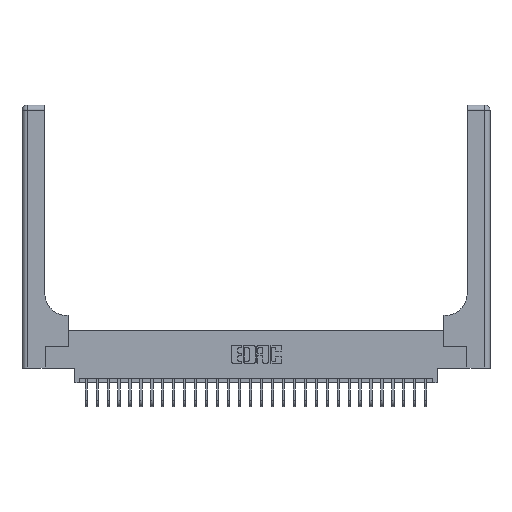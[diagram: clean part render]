
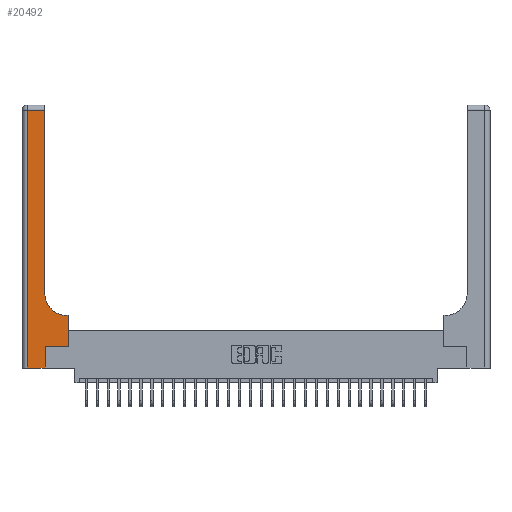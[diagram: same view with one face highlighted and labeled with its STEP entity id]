
A CAD part, top view. The second image highlights one B-rep face of the part: STEP entity #20492.
In plain terms, the highlighted planar face has unit normal (0, 0, 1).
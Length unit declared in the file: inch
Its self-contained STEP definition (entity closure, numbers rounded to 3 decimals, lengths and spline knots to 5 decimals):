
#137 = VERTEX_POINT ( 'NONE', #9777 ) ;
#267 = EDGE_LOOP ( 'NONE', ( #6003, #9272, #13486, #5783, #15114, #22827, #4643, #26591, #8260 ) ) ;
#576 = VERTEX_POINT ( 'NONE', #17336 ) ;
#908 = VECTOR ( 'NONE', #13147, 39.37008 ) ;
#946 = EDGE_CURVE ( 'NONE', #10002, #137, #17527, .T. ) ;
#1203 = CARTESIAN_POINT ( 'NONE',  ( 0.26, 2.94, 0.37 ) ) ;
#1216 = LINE ( 'NONE', #3422, #10927 ) ;
#1313 = PLANE ( 'NONE',  #22384 ) ;
#1940 = DIRECTION ( 'NONE',  ( -1., 0., 0. ) ) ;
#2091 = DIRECTION ( 'NONE',  ( 1., 0., 0. ) ) ;
#2163 = CARTESIAN_POINT ( 'NONE',  ( 0.51, 0.6, 0.37 ) ) ;
#2809 = LINE ( 'NONE', #24701, #23362 ) ;
#3154 = VECTOR ( 'NONE', #19565, 39.37008 ) ;
#3422 = CARTESIAN_POINT ( 'NONE',  ( 0., 0., 0.37 ) ) ;
#3699 = CARTESIAN_POINT ( 'NONE',  ( 0.528, 0.25, 0.37 ) ) ;
#4643 = ORIENTED_EDGE ( 'NONE', *, *, #16087, .T. ) ;
#5032 = VERTEX_POINT ( 'NONE', #20788 ) ;
#5483 = CARTESIAN_POINT ( 'NONE',  ( 0., 3., 0.37 ) ) ;
#5504 = DIRECTION ( 'NONE',  ( 1., 0., 0. ) ) ;
#5783 = ORIENTED_EDGE ( 'NONE', *, *, #23044, .T. ) ;
#5808 = CARTESIAN_POINT ( 'NONE',  ( 0.06, 2.94, 0.37 ) ) ;
#6003 = ORIENTED_EDGE ( 'NONE', *, *, #11436, .T. ) ;
#6098 = EDGE_CURVE ( 'NONE', #9677, #18002, #18338, .T. ) ;
#8156 = VERTEX_POINT ( 'NONE', #16663 ) ;
#8260 = ORIENTED_EDGE ( 'NONE', *, *, #946, .T. ) ;
#8759 = CARTESIAN_POINT ( 'NONE',  ( 0.265, 0.25, 0.37 ) ) ;
#8879 = LINE ( 'NONE', #11982, #19076 ) ;
#9272 = ORIENTED_EDGE ( 'NONE', *, *, #6098, .T. ) ;
#9677 = VERTEX_POINT ( 'NONE', #1203 ) ;
#9777 = CARTESIAN_POINT ( 'NONE',  ( 0.26, 0.85, 0.37 ) ) ;
#10002 = VERTEX_POINT ( 'NONE', #2163 ) ;
#10508 = VECTOR ( 'NONE', #18063, 39.37008 ) ;
#10825 = DIRECTION ( 'NONE',  ( 1., 0., 0. ) ) ;
#10927 = VECTOR ( 'NONE', #5504, 39.37008 ) ;
#11158 = VECTOR ( 'NONE', #10825, 39.37008 ) ;
#11436 = EDGE_CURVE ( 'NONE', #137, #9677, #22756, .T. ) ;
#11712 = DIRECTION ( 'NONE',  ( -1., 0., 0. ) ) ;
#11855 = EDGE_CURVE ( 'NONE', #18002, #8156, #2809, .T. ) ;
#11982 = CARTESIAN_POINT ( 'NONE',  ( 0.265, 0., 0.37 ) ) ;
#12412 = CARTESIAN_POINT ( 'NONE',  ( 0.51, 0.85, 0.37 ) ) ;
#12936 = VECTOR ( 'NONE', #1940, 39.37008 ) ;
#13139 = EDGE_CURVE ( 'NONE', #5032, #15210, #22009, .T. ) ;
#13147 = DIRECTION ( 'NONE',  ( 0., 1., 0. ) ) ;
#13486 = ORIENTED_EDGE ( 'NONE', *, *, #11855, .T. ) ;
#14031 = DIRECTION ( 'NONE',  ( 0., 1., 0. ) ) ;
#14447 = DIRECTION ( 'NONE',  ( 0., 0., -1. ) ) ;
#14766 = LINE ( 'NONE', #17543, #3154 ) ;
#15114 = ORIENTED_EDGE ( 'NONE', *, *, #25480, .T. ) ;
#15175 = CARTESIAN_POINT ( 'NONE',  ( 0.26, 3., 0.37 ) ) ;
#15210 = VERTEX_POINT ( 'NONE', #21229 ) ;
#16087 = EDGE_CURVE ( 'NONE', #15210, #576, #21337, .T. ) ;
#16350 = AXIS2_PLACEMENT_3D ( 'NONE', #12412, #14447, #2091 ) ;
#16663 = CARTESIAN_POINT ( 'NONE',  ( 0.06, 0., 0.37 ) ) ;
#17336 = CARTESIAN_POINT ( 'NONE',  ( 0.528, 0.6, 0.37 ) ) ;
#17527 = CIRCLE ( 'NONE', #16350, 0.25 ) ;
#17543 = CARTESIAN_POINT ( 'NONE',  ( 0.26, 0.6, 0.37 ) ) ;
#18002 = VERTEX_POINT ( 'NONE', #5808 ) ;
#18063 = DIRECTION ( 'NONE',  ( 0., 1., 0. ) ) ;
#18338 = LINE ( 'NONE', #18394, #12936 ) ;
#18394 = CARTESIAN_POINT ( 'NONE',  ( 0., 2.94, 0.37 ) ) ;
#19076 = VECTOR ( 'NONE', #14031, 39.37008 ) ;
#19565 = DIRECTION ( 'NONE',  ( -1., 0., 0. ) ) ;
#20053 = VERTEX_POINT ( 'NONE', #20218 ) ;
#20218 = CARTESIAN_POINT ( 'NONE',  ( 0.265, 0., 0.37 ) ) ;
#20492 = ADVANCED_FACE ( 'NONE', ( #26565 ), #1313, .F. ) ;
#20686 = DIRECTION ( 'NONE',  ( 0., -1., 0. ) ) ;
#20788 = CARTESIAN_POINT ( 'NONE',  ( 0.265, 0.25, 0.37 ) ) ;
#21229 = CARTESIAN_POINT ( 'NONE',  ( 0.528, 0.25, 0.37 ) ) ;
#21337 = LINE ( 'NONE', #3699, #10508 ) ;
#22009 = LINE ( 'NONE', #8759, #11158 ) ;
#22384 = AXIS2_PLACEMENT_3D ( 'NONE', #5483, #23919, #11712 ) ;
#22756 = LINE ( 'NONE', #15175, #908 ) ;
#22827 = ORIENTED_EDGE ( 'NONE', *, *, #13139, .T. ) ;
#22932 = EDGE_CURVE ( 'NONE', #576, #10002, #14766, .T. ) ;
#23044 = EDGE_CURVE ( 'NONE', #8156, #20053, #1216, .T. ) ;
#23362 = VECTOR ( 'NONE', #20686, 39.37008 ) ;
#23919 = DIRECTION ( 'NONE',  ( 0., 0., -1. ) ) ;
#24701 = CARTESIAN_POINT ( 'NONE',  ( 0.06, 3., 0.37 ) ) ;
#25480 = EDGE_CURVE ( 'NONE', #20053, #5032, #8879, .T. ) ;
#26565 = FACE_OUTER_BOUND ( 'NONE', #267, .T. ) ;
#26591 = ORIENTED_EDGE ( 'NONE', *, *, #22932, .T. ) ;
